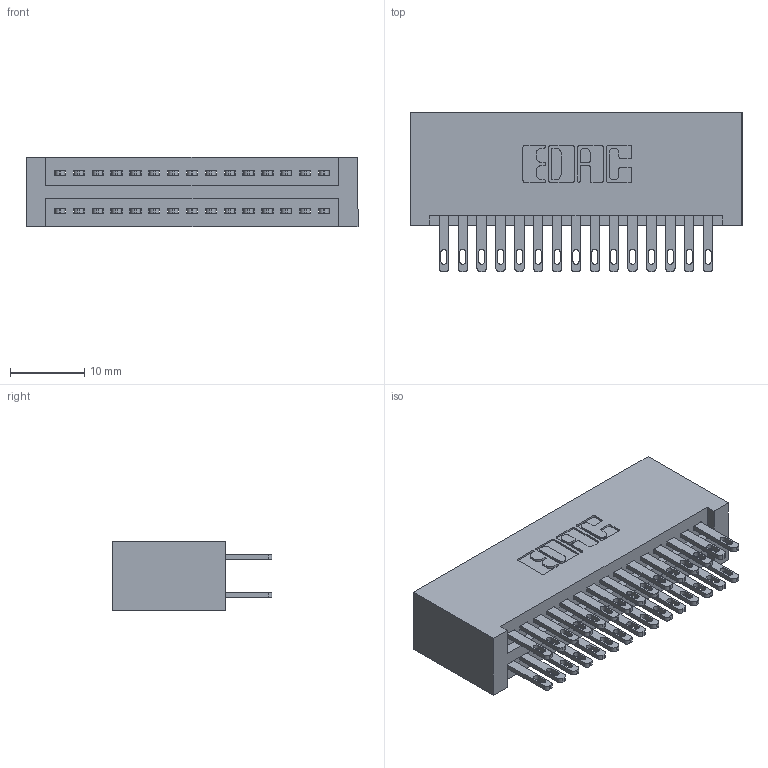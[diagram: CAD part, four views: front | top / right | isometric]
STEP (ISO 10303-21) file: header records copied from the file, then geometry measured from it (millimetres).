
FILE_DESCRIPTION (( 'STEP AP203' ), '1' );
FILE_NAME ('895-030-500-201.STEP', '2020-09-25T17:33:56', ( '' ), ( '' ), 'SwSTEP 2.0', 'SolidWorks 2020', '' );
FILE_SCHEMA (( 'CONFIG_CONTROL_DESIGN' ));
Length unit declared in the file: inch
Products named in the file (3): 845 Part_No Mounting Lugs; 345-292-001_345-293-100; 895-030-500-201
Assembly tree (31 placements, depth 2):
  895-030-500-201
    845 Part_No Mounting Lugs
    345-292-001_345-293-100  x30
Bounding box: 44.7 x 21.51 x 9.4 mm (x, y, z)
Volume: 4799.6 mm3; surface area: 7180.9 mm2
Topology: 31 solids, 31 shells, 1498 faces, 4547 edges, 3030 vertices
Faces by surface type: plane 886, cylinder 612
Entity records: 15057 total; most frequent: CARTESIAN_POINT 2548, ORIENTED_EDGE 2482, DIRECTION 2277, EDGE_CURVE 1241, VECTOR 1053, LINE 1053, VERTEX_POINT 826, AXIS2_PLACEMENT_3D 612
